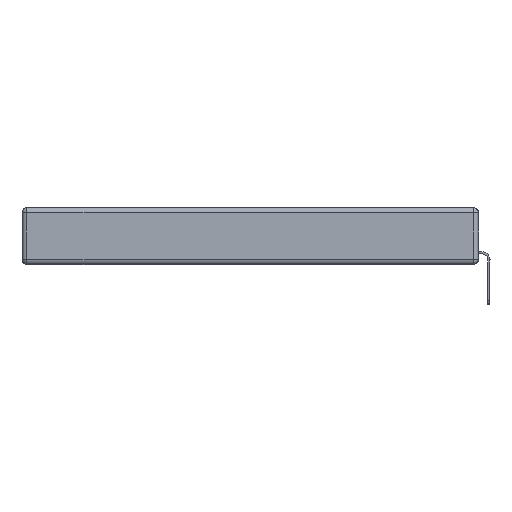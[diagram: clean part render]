
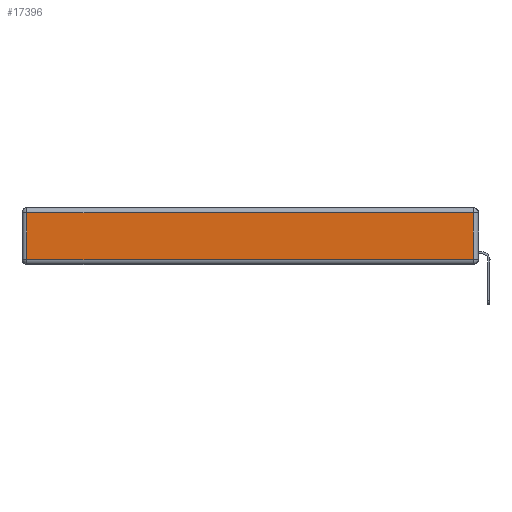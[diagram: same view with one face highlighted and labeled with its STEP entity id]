
A CAD part, left-side view. The second image highlights one B-rep face of the part: STEP entity #17396.
In plain terms, the highlighted planar face has unit normal (-1, 0, 0).
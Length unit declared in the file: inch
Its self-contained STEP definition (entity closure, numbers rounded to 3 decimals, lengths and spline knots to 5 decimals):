
#99 = ORIENTED_EDGE ( 'NONE', *, *, #4218, .T. ) ;
#1204 = VECTOR ( 'NONE', #21207, 39.37008 ) ;
#2564 = ORIENTED_EDGE ( 'NONE', *, *, #21873, .T. ) ;
#4218 = EDGE_CURVE ( 'NONE', #18569, #8059, #6241, .T. ) ;
#4247 = CARTESIAN_POINT ( 'NONE',  ( 0., 0., -0.343 ) ) ;
#4855 = ORIENTED_EDGE ( 'NONE', *, *, #20877, .T. ) ;
#6049 = DIRECTION ( 'NONE',  ( 0., 1., 0. ) ) ;
#6124 = CARTESIAN_POINT ( 'NONE',  ( 0., 0.03, -0.03 ) ) ;
#6241 = LINE ( 'NONE', #13737, #1204 ) ;
#7564 = EDGE_LOOP ( 'NONE', ( #99, #7992, #2564, #4855 ) ) ;
#7656 = CARTESIAN_POINT ( 'NONE',  ( 0., 2.72, -0.03 ) ) ;
#7771 = DIRECTION ( 'NONE',  ( 0., 0., 1. ) ) ;
#7992 = ORIENTED_EDGE ( 'NONE', *, *, #12919, .T. ) ;
#8059 = VERTEX_POINT ( 'NONE', #22102 ) ;
#8146 = DIRECTION ( 'NONE',  ( -1., 0., 0. ) ) ;
#8262 = VECTOR ( 'NONE', #8886, 39.37008 ) ;
#8886 = DIRECTION ( 'NONE',  ( 0., 0., 1. ) ) ;
#9668 = VECTOR ( 'NONE', #6049, 39.37008 ) ;
#11203 = PLANE ( 'NONE',  #15382 ) ;
#12373 = VERTEX_POINT ( 'NONE', #6124 ) ;
#12919 = EDGE_CURVE ( 'NONE', #8059, #12373, #16359, .T. ) ;
#13737 = CARTESIAN_POINT ( 'NONE',  ( 0., 0., -0.313 ) ) ;
#15382 = AXIS2_PLACEMENT_3D ( 'NONE', #4247, #8146, #7771 ) ;
#15791 = CARTESIAN_POINT ( 'NONE',  ( 0., 0.03, -0.343 ) ) ;
#16359 = LINE ( 'NONE', #15791, #8262 ) ;
#17045 = LINE ( 'NONE', #20844, #20594 ) ;
#17396 = ADVANCED_FACE ( 'NONE', ( #20528 ), #11203, .T. ) ;
#17415 = DIRECTION ( 'NONE',  ( 0., 0., -1. ) ) ;
#17446 = LINE ( 'NONE', #18907, #9668 ) ;
#18569 = VERTEX_POINT ( 'NONE', #18686 ) ;
#18686 = CARTESIAN_POINT ( 'NONE',  ( 0., 2.72, -0.313 ) ) ;
#18692 = VERTEX_POINT ( 'NONE', #7656 ) ;
#18907 = CARTESIAN_POINT ( 'NONE',  ( 0., 2.75, -0.03 ) ) ;
#20528 = FACE_OUTER_BOUND ( 'NONE', #7564, .T. ) ;
#20594 = VECTOR ( 'NONE', #17415, 39.37008 ) ;
#20844 = CARTESIAN_POINT ( 'NONE',  ( 0., 2.72, -0.343 ) ) ;
#20877 = EDGE_CURVE ( 'NONE', #18692, #18569, #17045, .T. ) ;
#21207 = DIRECTION ( 'NONE',  ( 0., -1., 0. ) ) ;
#21873 = EDGE_CURVE ( 'NONE', #12373, #18692, #17446, .T. ) ;
#22102 = CARTESIAN_POINT ( 'NONE',  ( 0., 0.03, -0.313 ) ) ;
